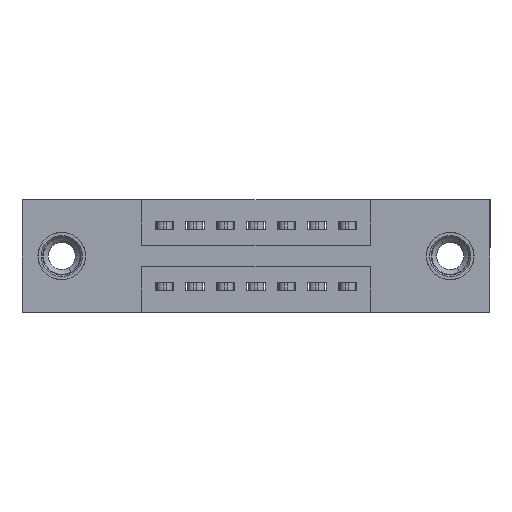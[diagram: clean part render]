
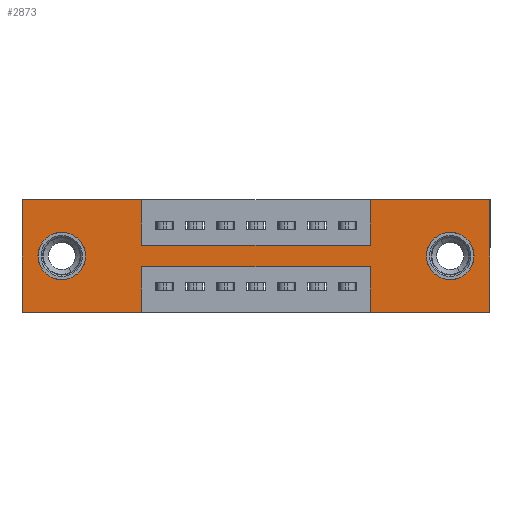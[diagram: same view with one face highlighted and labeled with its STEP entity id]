
A CAD part, front view. The second image highlights one B-rep face of the part: STEP entity #2873.
In plain terms, the highlighted planar face has unit normal (0, -1, 0).
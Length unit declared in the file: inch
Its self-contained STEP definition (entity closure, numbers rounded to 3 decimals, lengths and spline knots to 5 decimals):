
#9 = EDGE_CURVE ( 'NONE', #9971, #4291, #4170, .T. ) ;
#28 = CARTESIAN_POINT ( 'NONE',  ( 1.405, 0., -0.263 ) ) ;
#87 = CARTESIAN_POINT ( 'NONE',  ( 0., 0., 0. ) ) ;
#226 = EDGE_CURVE ( 'NONE', #2663, #14698, #2721, .T. ) ;
#267 = CARTESIAN_POINT ( 'NONE',  ( 0.3925, 0., -0.37 ) ) ;
#296 = DIRECTION ( 'NONE',  ( -1., 0., 0. ) ) ;
#335 = LINE ( 'NONE', #6067, #11827 ) ;
#352 = EDGE_CURVE ( 'NONE', #4710, #4523, #14668, .T. ) ;
#456 = DIRECTION ( 'NONE',  ( 0., 0., 1. ) ) ;
#544 = CARTESIAN_POINT ( 'NONE',  ( 0., 0., -0.37 ) ) ;
#623 = DIRECTION ( 'NONE',  ( 0., 1., 0. ) ) ;
#704 = DIRECTION ( 'NONE',  ( 0., -1., 0. ) ) ;
#917 = VERTEX_POINT ( 'NONE', #3265 ) ;
#920 = EDGE_CURVE ( 'NONE', #4053, #7540, #12091, .T. ) ;
#964 = VECTOR ( 'NONE', #13680, 39.37008 ) ;
#966 = ORIENTED_EDGE ( 'NONE', *, *, #10342, .F. ) ;
#1087 = FACE_OUTER_BOUND ( 'NONE', #14634, .T. ) ;
#1186 = CARTESIAN_POINT ( 'NONE',  ( 1.535, 0., -0.37 ) ) ;
#1411 = CARTESIAN_POINT ( 'NONE',  ( 1.535, 0., 0. ) ) ;
#1570 = ORIENTED_EDGE ( 'NONE', *, *, #13981, .F. ) ;
#1736 = CARTESIAN_POINT ( 'NONE',  ( 0., 0., -0.37 ) ) ;
#1775 = AXIS2_PLACEMENT_3D ( 'NONE', #1736, #704, #14335 ) ;
#1842 = VECTOR ( 'NONE', #2381, 39.37008 ) ;
#1866 = EDGE_CURVE ( 'NONE', #14698, #2663, #10972, .T. ) ;
#2030 = CARTESIAN_POINT ( 'NONE',  ( 1.1425, 0., -0.15 ) ) ;
#2111 = VECTOR ( 'NONE', #13640, 39.37008 ) ;
#2142 = EDGE_CURVE ( 'NONE', #6926, #10095, #4104, .T. ) ;
#2159 = CARTESIAN_POINT ( 'NONE',  ( 1.1425, 0., -0.22 ) ) ;
#2381 = DIRECTION ( 'NONE',  ( 0., 0., 1. ) ) ;
#2574 = CARTESIAN_POINT ( 'NONE',  ( 0.13, 0., -0.263 ) ) ;
#2663 = VERTEX_POINT ( 'NONE', #4600 ) ;
#2721 = CIRCLE ( 'NONE', #11336, 0.078 ) ;
#2866 = EDGE_CURVE ( 'NONE', #10095, #5315, #9085, .T. ) ;
#2873 = ADVANCED_FACE ( 'NONE', ( #11126, #13841, #1087 ), #13316, .T. ) ;
#2878 = AXIS2_PLACEMENT_3D ( 'NONE', #14563, #7500, #12216 ) ;
#2897 = CARTESIAN_POINT ( 'NONE',  ( 0., 0., -0.37 ) ) ;
#3265 = CARTESIAN_POINT ( 'NONE',  ( 0.3925, 0., -0.15 ) ) ;
#3334 = ORIENTED_EDGE ( 'NONE', *, *, #1866, .T. ) ;
#3372 = CARTESIAN_POINT ( 'NONE',  ( 1.535, 0., 0. ) ) ;
#3420 = ORIENTED_EDGE ( 'NONE', *, *, #352, .F. ) ;
#3466 = DIRECTION ( 'NONE',  ( 0., 0., -1. ) ) ;
#3494 = LINE ( 'NONE', #7626, #11443 ) ;
#3515 = LINE ( 'NONE', #10116, #2111 ) ;
#3887 = DIRECTION ( 'NONE',  ( -1., 0., 0. ) ) ;
#4053 = VERTEX_POINT ( 'NONE', #14664 ) ;
#4074 = DIRECTION ( 'NONE',  ( 0., 0., -1. ) ) ;
#4104 = LINE ( 'NONE', #13349, #7868 ) ;
#4170 = LINE ( 'NONE', #2897, #4887 ) ;
#4291 = VERTEX_POINT ( 'NONE', #14045 ) ;
#4392 = DIRECTION ( 'NONE',  ( 0., 0., 1. ) ) ;
#4468 = ORIENTED_EDGE ( 'NONE', *, *, #9758, .T. ) ;
#4523 = VERTEX_POINT ( 'NONE', #1411 ) ;
#4549 = VERTEX_POINT ( 'NONE', #2574 ) ;
#4558 = DIRECTION ( 'NONE',  ( 1., 0., 0. ) ) ;
#4600 = CARTESIAN_POINT ( 'NONE',  ( 1.405, 0., -0.107 ) ) ;
#4630 = CARTESIAN_POINT ( 'NONE',  ( 0.3925, 0., -0.22 ) ) ;
#4710 = VERTEX_POINT ( 'NONE', #9555 ) ;
#4887 = VECTOR ( 'NONE', #3887, 39.37008 ) ;
#4897 = ORIENTED_EDGE ( 'NONE', *, *, #10645, .F. ) ;
#5202 = ORIENTED_EDGE ( 'NONE', *, *, #14349, .F. ) ;
#5315 = VERTEX_POINT ( 'NONE', #6369 ) ;
#5407 = ORIENTED_EDGE ( 'NONE', *, *, #6965, .F. ) ;
#5542 = DIRECTION ( 'NONE',  ( 0., 1., 0. ) ) ;
#5544 = ORIENTED_EDGE ( 'NONE', *, *, #10894, .T. ) ;
#5553 = LINE ( 'NONE', #11733, #9812 ) ;
#5912 = ORIENTED_EDGE ( 'NONE', *, *, #2142, .F. ) ;
#6067 = CARTESIAN_POINT ( 'NONE',  ( 0.3925, 0., 0. ) ) ;
#6313 = CARTESIAN_POINT ( 'NONE',  ( 0.13, 0., -0.185 ) ) ;
#6369 = CARTESIAN_POINT ( 'NONE',  ( 0., 0., -0.37 ) ) ;
#6437 = CIRCLE ( 'NONE', #6566, 0.078 ) ;
#6566 = AXIS2_PLACEMENT_3D ( 'NONE', #11164, #5542, #13472 ) ;
#6631 = CARTESIAN_POINT ( 'NONE',  ( 1.1425, 0., -0.37 ) ) ;
#6795 = EDGE_CURVE ( 'NONE', #4291, #13671, #7208, .T. ) ;
#6796 = VECTOR ( 'NONE', #12137, 39.37008 ) ;
#6926 = VERTEX_POINT ( 'NONE', #4630 ) ;
#6965 = EDGE_CURVE ( 'NONE', #5315, #4053, #7888, .T. ) ;
#7040 = AXIS2_PLACEMENT_3D ( 'NONE', #6313, #10980, #456 ) ;
#7208 = LINE ( 'NONE', #6631, #12629 ) ;
#7500 = DIRECTION ( 'NONE',  ( 0., 1., 0. ) ) ;
#7540 = VERTEX_POINT ( 'NONE', #12845 ) ;
#7626 = CARTESIAN_POINT ( 'NONE',  ( 0.3925, 0., -0.15 ) ) ;
#7868 = VECTOR ( 'NONE', #4074, 39.37008 ) ;
#7888 = LINE ( 'NONE', #11105, #1842 ) ;
#8340 = VECTOR ( 'NONE', #3466, 39.37008 ) ;
#8973 = CARTESIAN_POINT ( 'NONE',  ( 0., 0., 0. ) ) ;
#9085 = LINE ( 'NONE', #544, #6796 ) ;
#9149 = VECTOR ( 'NONE', #4558, 39.37008 ) ;
#9493 = DIRECTION ( 'NONE',  ( 0., 0., -1. ) ) ;
#9555 = CARTESIAN_POINT ( 'NONE',  ( 1.1425, 0., 0. ) ) ;
#9691 = CARTESIAN_POINT ( 'NONE',  ( 1.405, 0., -0.185 ) ) ;
#9758 = EDGE_CURVE ( 'NONE', #4549, #9833, #6437, .T. ) ;
#9762 = DIRECTION ( 'NONE',  ( 1., 0., 0. ) ) ;
#9812 = VECTOR ( 'NONE', #296, 39.37008 ) ;
#9833 = VERTEX_POINT ( 'NONE', #10048 ) ;
#9845 = VERTEX_POINT ( 'NONE', #2030 ) ;
#9971 = VERTEX_POINT ( 'NONE', #1186 ) ;
#10048 = CARTESIAN_POINT ( 'NONE',  ( 0.13, 0., -0.107 ) ) ;
#10095 = VERTEX_POINT ( 'NONE', #267 ) ;
#10116 = CARTESIAN_POINT ( 'NONE',  ( 1.1425, 0., 0. ) ) ;
#10342 = EDGE_CURVE ( 'NONE', #917, #9845, #3494, .T. ) ;
#10645 = EDGE_CURVE ( 'NONE', #4523, #9971, #13460, .T. ) ;
#10894 = EDGE_CURVE ( 'NONE', #9833, #4549, #11975, .T. ) ;
#10972 = CIRCLE ( 'NONE', #2878, 0.078 ) ;
#10980 = DIRECTION ( 'NONE',  ( 0., 1., 0. ) ) ;
#11105 = CARTESIAN_POINT ( 'NONE',  ( 0., 0., 0. ) ) ;
#11126 = FACE_BOUND ( 'NONE', #11195, .T. ) ;
#11164 = CARTESIAN_POINT ( 'NONE',  ( 0.13, 0., -0.185 ) ) ;
#11195 = EDGE_LOOP ( 'NONE', ( #12508, #3334 ) ) ;
#11336 = AXIS2_PLACEMENT_3D ( 'NONE', #9691, #623, #13348 ) ;
#11443 = VECTOR ( 'NONE', #9762, 39.37008 ) ;
#11733 = CARTESIAN_POINT ( 'NONE',  ( 0.3925, 0., -0.22 ) ) ;
#11827 = VECTOR ( 'NONE', #9493, 39.37008 ) ;
#11914 = ORIENTED_EDGE ( 'NONE', *, *, #14050, .F. ) ;
#11975 = CIRCLE ( 'NONE', #7040, 0.078 ) ;
#12091 = LINE ( 'NONE', #8973, #964 ) ;
#12137 = DIRECTION ( 'NONE',  ( -1., 0., 0. ) ) ;
#12216 = DIRECTION ( 'NONE',  ( 0., 0., -1. ) ) ;
#12508 = ORIENTED_EDGE ( 'NONE', *, *, #226, .T. ) ;
#12538 = ORIENTED_EDGE ( 'NONE', *, *, #6795, .F. ) ;
#12629 = VECTOR ( 'NONE', #4392, 39.37008 ) ;
#12730 = ORIENTED_EDGE ( 'NONE', *, *, #2866, .F. ) ;
#12845 = CARTESIAN_POINT ( 'NONE',  ( 0.3925, 0., 0. ) ) ;
#13316 = PLANE ( 'NONE',  #1775 ) ;
#13348 = DIRECTION ( 'NONE',  ( 0., 0., -1. ) ) ;
#13349 = CARTESIAN_POINT ( 'NONE',  ( 0.3925, 0., -0.37 ) ) ;
#13460 = LINE ( 'NONE', #3372, #8340 ) ;
#13472 = DIRECTION ( 'NONE',  ( 0., 0., 1. ) ) ;
#13640 = DIRECTION ( 'NONE',  ( 0., 0., 1. ) ) ;
#13671 = VERTEX_POINT ( 'NONE', #2159 ) ;
#13680 = DIRECTION ( 'NONE',  ( 1., 0., 0. ) ) ;
#13841 = FACE_BOUND ( 'NONE', #13857, .T. ) ;
#13857 = EDGE_LOOP ( 'NONE', ( #5544, #4468 ) ) ;
#13981 = EDGE_CURVE ( 'NONE', #7540, #917, #335, .T. ) ;
#14045 = CARTESIAN_POINT ( 'NONE',  ( 1.1425, 0., -0.37 ) ) ;
#14050 = EDGE_CURVE ( 'NONE', #9845, #4710, #3515, .T. ) ;
#14335 = DIRECTION ( 'NONE',  ( 0., 0., -1. ) ) ;
#14349 = EDGE_CURVE ( 'NONE', #13671, #6926, #5553, .T. ) ;
#14563 = CARTESIAN_POINT ( 'NONE',  ( 1.405, 0., -0.185 ) ) ;
#14634 = EDGE_LOOP ( 'NONE', ( #5912, #5202, #12538, #14791, #4897, #3420, #11914, #966, #1570, #14706, #5407, #12730 ) ) ;
#14664 = CARTESIAN_POINT ( 'NONE',  ( 0., 0., 0. ) ) ;
#14668 = LINE ( 'NONE', #87, #9149 ) ;
#14698 = VERTEX_POINT ( 'NONE', #28 ) ;
#14706 = ORIENTED_EDGE ( 'NONE', *, *, #920, .F. ) ;
#14791 = ORIENTED_EDGE ( 'NONE', *, *, #9, .F. ) ;
